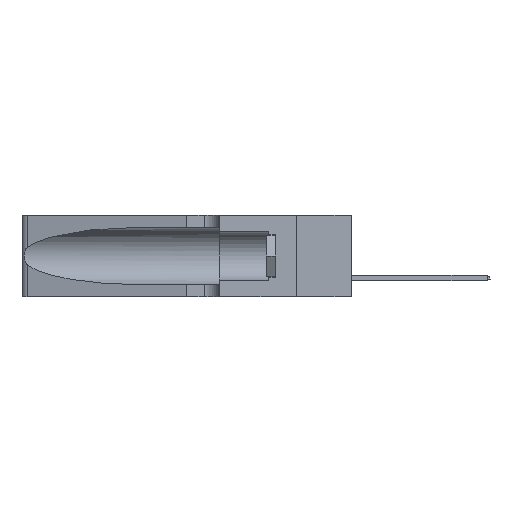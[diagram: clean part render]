
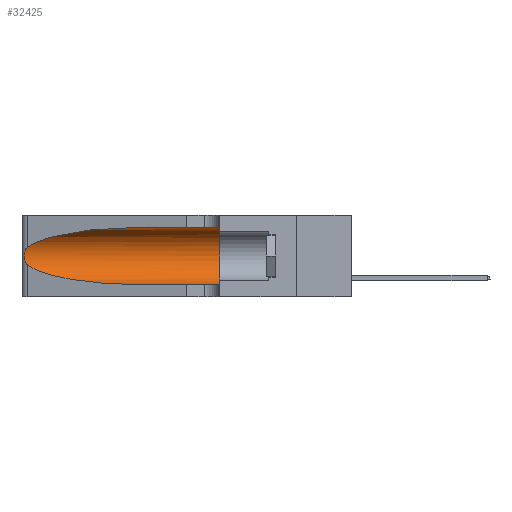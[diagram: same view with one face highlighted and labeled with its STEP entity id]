
A CAD part, left-side view. The second image highlights one B-rep face of the part: STEP entity #32425.
In plain terms, the highlighted cylindrical face has radius 3.308 mm (diameter 6.617 mm), a partial arc.
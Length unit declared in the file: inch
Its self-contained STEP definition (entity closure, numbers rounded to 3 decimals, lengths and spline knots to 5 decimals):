
#864 = EDGE_CURVE ( 'NONE', #32767, #20015, #16046, .T. ) ;
#976 = EDGE_CURVE ( 'NONE', #30201, #32693, #6914, .T. ) ;
#1015 = LINE ( 'NONE', #24285, #8672 ) ;
#1305 = DIRECTION ( 'NONE',  ( 0., 0., 1. ) ) ;
#1365 =( BOUNDED_CURVE ( )  B_SPLINE_CURVE ( 3, ( #5213, #23368, #28387, #10419 ),
 .UNSPECIFIED., .F., .T. ) 
 B_SPLINE_CURVE_WITH_KNOTS ( ( 4, 4 ),
 ( 3.44316, 4.71239 ),
 .UNSPECIFIED. ) 
 CURVE ( )  GEOMETRIC_REPRESENTATION_ITEM ( )  RATIONAL_B_SPLINE_CURVE ( ( 1., 0.87, 0.87, 1. ) ) 
 REPRESENTATION_ITEM ( '' )  );
#2832 = ORIENTED_EDGE ( 'NONE', *, *, #976, .T. ) ;
#2868 = FACE_OUTER_BOUND ( 'NONE', #22747, .T. ) ;
#3371 = VERTEX_POINT ( 'NONE', #18829 ) ;
#4373 = ORIENTED_EDGE ( 'NONE', *, *, #29695, .F. ) ;
#5213 = CARTESIAN_POINT ( 'NONE',  ( 0.25487, 1.22718, 0.14631 ) ) ;
#5545 = ORIENTED_EDGE ( 'NONE', *, *, #864, .T. ) ;
#6678 = CARTESIAN_POINT ( 'NONE',  ( 0.25555, 1.22994, 0.2215 ) ) ;
#6914 = B_SPLINE_CURVE_WITH_KNOTS ( 'NONE', 3,
 ( #29937, #6678, #11770, #22350, #11888, #9628, #27491, #30040, #32171, #19458, #24596, #9281, #14420, #14870 ),
 .UNSPECIFIED., .F., .F.,
 ( 4, 2, 2, 2, 2, 2, 4 ),
 ( 0., 0.00027, 0.00053, 0.00107, 0.0016, 0.00187, 0.00214 ),
 .UNSPECIFIED. ) ;
#7050 = DIRECTION ( 'NONE',  ( 0., -1., 0. ) ) ;
#7595 = DIRECTION ( 'NONE',  ( 0., -1., 0. ) ) ;
#8672 = VECTOR ( 'NONE', #7050, 39.37008 ) ;
#9281 = CARTESIAN_POINT ( 'NONE',  ( 0.25639, 1.23186, 0.15144 ) ) ;
#9470 = AXIS2_PLACEMENT_3D ( 'NONE', #12790, #7595, #20258 ) ;
#9628 = CARTESIAN_POINT ( 'NONE',  ( 0.26018, 1.23835, 0.19895 ) ) ;
#10008 = EDGE_CURVE ( 'NONE', #32693, #32767, #1365, .T. ) ;
#10419 = CARTESIAN_POINT ( 'NONE',  ( 0.1305, 0.72297, 0.05475 ) ) ;
#10904 = ORIENTED_EDGE ( 'NONE', *, *, #18887, .F. ) ;
#11410 = CARTESIAN_POINT ( 'NONE',  ( 0.25487, 1.22718, 0.22369 ) ) ;
#11770 = CARTESIAN_POINT ( 'NONE',  ( 0.25639, 1.23184, 0.21858 ) ) ;
#11888 = CARTESIAN_POINT ( 'NONE',  ( 0.25854, 1.2359, 0.20912 ) ) ;
#12304 = CIRCLE ( 'NONE', #13768, 0.13025 ) ;
#12790 = CARTESIAN_POINT ( 'NONE',  ( 0.1305, 1.61858, 0.185 ) ) ;
#13462 = CARTESIAN_POINT ( 'NONE',  ( 0.1305, 0.72297, 0.31525 ) ) ;
#13768 = AXIS2_PLACEMENT_3D ( 'NONE', #14122, #18907, #1305 ) ;
#14122 = CARTESIAN_POINT ( 'NONE',  ( 0.1305, 0.35, 0.185 ) ) ;
#14420 = CARTESIAN_POINT ( 'NONE',  ( 0.25555, 1.22993, 0.14849 ) ) ;
#14812 = VECTOR ( 'NONE', #15906, 39.37008 ) ;
#14870 = CARTESIAN_POINT ( 'NONE',  ( 0.25487, 1.22718, 0.14631 ) ) ;
#15906 = DIRECTION ( 'NONE',  ( 0., -1., 0. ) ) ;
#16046 = LINE ( 'NONE', #28631, #14812 ) ;
#16315 = CARTESIAN_POINT ( 'NONE',  ( 0.2373, 1.15595, 0.28018 ) ) ;
#18761 = CARTESIAN_POINT ( 'NONE',  ( 0.25487, 1.22718, 0.22369 ) ) ;
#18829 = CARTESIAN_POINT ( 'NONE',  ( 0.1305, 0.72297, 0.31525 ) ) ;
#18887 = EDGE_CURVE ( 'NONE', #22412, #20015, #12304, .T. ) ;
#18907 = DIRECTION ( 'NONE',  ( 0., 1., 0. ) ) ;
#19458 = CARTESIAN_POINT ( 'NONE',  ( 0.25856, 1.23593, 0.16098 ) ) ;
#20015 = VERTEX_POINT ( 'NONE', #25598 ) ;
#20258 = DIRECTION ( 'NONE',  ( 0., 0., -1. ) ) ;
#20913 = CARTESIAN_POINT ( 'NONE',  ( 0.18966, 0.96281, 0.31525 ) ) ;
#21760 = CARTESIAN_POINT ( 'NONE',  ( 0.1305, 0.72297, 0.05475 ) ) ;
#22350 = CARTESIAN_POINT ( 'NONE',  ( 0.25787, 1.23484, 0.2124 ) ) ;
#22412 = VERTEX_POINT ( 'NONE', #24114 ) ;
#22747 = EDGE_LOOP ( 'NONE', ( #25805, #2832, #32406, #5545, #10904, #4373 ) ) ;
#23368 = CARTESIAN_POINT ( 'NONE',  ( 0.2373, 1.15595, 0.08982 ) ) ;
#23805 = CARTESIAN_POINT ( 'NONE',  ( 0.25487, 1.22718, 0.14631 ) ) ;
#24114 = CARTESIAN_POINT ( 'NONE',  ( 0.1305, 0.35, 0.31525 ) ) ;
#24285 = CARTESIAN_POINT ( 'NONE',  ( 0.1305, 1.61858, 0.31525 ) ) ;
#24596 = CARTESIAN_POINT ( 'NONE',  ( 0.25789, 1.23486, 0.15765 ) ) ;
#25598 = CARTESIAN_POINT ( 'NONE',  ( 0.1305, 0.35, 0.05475 ) ) ;
#25805 = ORIENTED_EDGE ( 'NONE', *, *, #30148, .T. ) ;
#27256 = CYLINDRICAL_SURFACE ( 'NONE', #9470, 0.13025 ) ;
#27491 = CARTESIAN_POINT ( 'NONE',  ( 0.26075, 1.23896, 0.19203 ) ) ;
#28387 = CARTESIAN_POINT ( 'NONE',  ( 0.18966, 0.96281, 0.05475 ) ) ;
#28631 = CARTESIAN_POINT ( 'NONE',  ( 0.1305, 1.61858, 0.05475 ) ) ;
#29083 =( BOUNDED_CURVE ( )  B_SPLINE_CURVE ( 3, ( #13462, #20913, #16315, #11410 ),
 .UNSPECIFIED., .F., .F. ) 
 B_SPLINE_CURVE_WITH_KNOTS ( ( 4, 4 ),
 ( 1.5708, 2.84003 ),
 .UNSPECIFIED. ) 
 CURVE ( )  GEOMETRIC_REPRESENTATION_ITEM ( )  RATIONAL_B_SPLINE_CURVE ( ( 1., 0.87, 0.87, 1. ) ) 
 REPRESENTATION_ITEM ( '' )  );
#29695 = EDGE_CURVE ( 'NONE', #3371, #22412, #1015, .T. ) ;
#29937 = CARTESIAN_POINT ( 'NONE',  ( 0.25487, 1.22718, 0.22369 ) ) ;
#30040 = CARTESIAN_POINT ( 'NONE',  ( 0.26075, 1.23896, 0.178 ) ) ;
#30148 = EDGE_CURVE ( 'NONE', #3371, #30201, #29083, .T. ) ;
#30201 = VERTEX_POINT ( 'NONE', #18761 ) ;
#32171 = CARTESIAN_POINT ( 'NONE',  ( 0.26017, 1.23833, 0.17102 ) ) ;
#32406 = ORIENTED_EDGE ( 'NONE', *, *, #10008, .T. ) ;
#32425 = ADVANCED_FACE ( 'NONE', ( #2868 ), #27256, .F. ) ;
#32693 = VERTEX_POINT ( 'NONE', #23805 ) ;
#32767 = VERTEX_POINT ( 'NONE', #21760 ) ;
